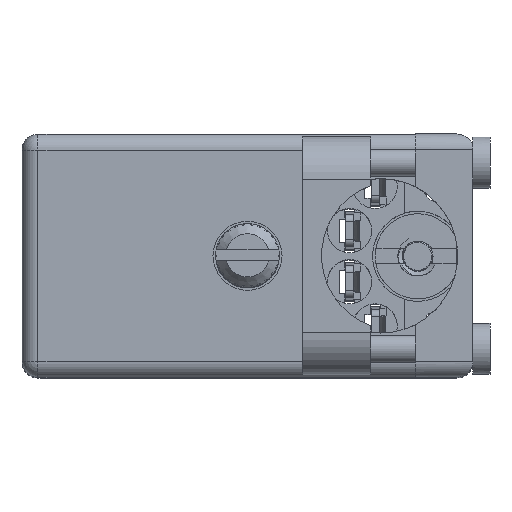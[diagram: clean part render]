
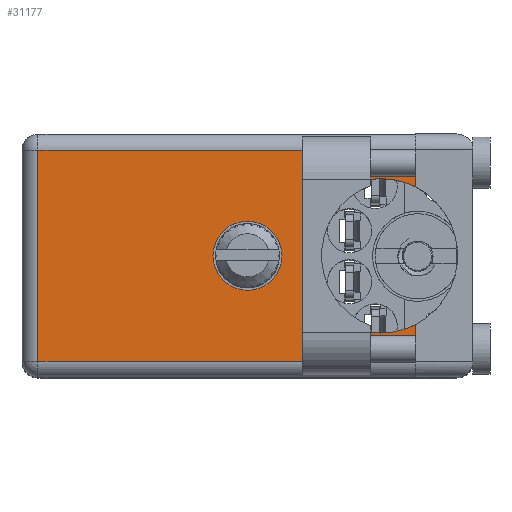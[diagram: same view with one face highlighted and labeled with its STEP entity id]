
A CAD part, top view. The second image highlights one B-rep face of the part: STEP entity #31177.
In plain terms, the highlighted face is planar.
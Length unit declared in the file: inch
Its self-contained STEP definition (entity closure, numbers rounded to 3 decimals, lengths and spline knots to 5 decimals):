
#836 = VERTEX_POINT ( 'NONE', #193161 ) ;
#1619 = CARTESIAN_POINT ( 'NONE',  ( 1.155, 0.906, -0.15471 ) ) ;
#1675 = CARTESIAN_POINT ( 'NONE',  ( 1.155, 0.906, -0.668 ) ) ;
#5758 = DIRECTION ( 'NONE',  ( 0., 0., 1. ) ) ;
#6183 = CARTESIAN_POINT ( 'NONE',  ( 1.155, 0.906, 0. ) ) ;
#8776 = CARTESIAN_POINT ( 'NONE',  ( 1.053, 0.906, -0.5845 ) ) ;
#14136 = DIRECTION ( 'NONE',  ( 0., 1., 0. ) ) ;
#14505 = ORIENTED_EDGE ( 'NONE', *, *, #89355, .T. ) ;
#15905 = VERTEX_POINT ( 'NONE', #1619 ) ;
#20903 = DIRECTION ( 'NONE',  ( 0., 0., 1. ) ) ;
#24156 = VECTOR ( 'NONE', #189563, 39.37008 ) ;
#27023 = ORIENTED_EDGE ( 'NONE', *, *, #172200, .F. ) ;
#27527 = CARTESIAN_POINT ( 'NONE',  ( 1.155, 0.906, -0.047 ) ) ;
#28790 = CARTESIAN_POINT ( 'NONE',  ( 1.053, 0.906, -0.3575 ) ) ;
#31177 = ADVANCED_FACE ( 'NONE', ( #39452, #183516 ), #131591, .T. ) ;
#31375 = EDGE_CURVE ( 'NONE', #836, #15905, #49074, .T. ) ;
#31876 = ORIENTED_EDGE ( 'NONE', *, *, #49957, .F. ) ;
#34957 = DIRECTION ( 'NONE',  ( 0., 1., 0. ) ) ;
#35433 = CIRCLE ( 'NONE', #134394, 0.227 ) ;
#38335 = DIRECTION ( 'NONE',  ( 0., 1., 0. ) ) ;
#39452 = FACE_OUTER_BOUND ( 'NONE', #113883, .T. ) ;
#41365 = VERTEX_POINT ( 'NONE', #27527 ) ;
#45925 = VECTOR ( 'NONE', #118477, 39.37008 ) ;
#46874 = VERTEX_POINT ( 'NONE', #136284 ) ;
#47317 = ORIENTED_EDGE ( 'NONE', *, *, #54023, .F. ) ;
#48261 = CARTESIAN_POINT ( 'NONE',  ( 1.053, 0.906, -0.3575 ) ) ;
#49074 = CIRCLE ( 'NONE', #132033, 0.227 ) ;
#49957 = EDGE_CURVE ( 'NONE', #15905, #41365, #113801, .T. ) ;
#51064 = CIRCLE ( 'NONE', #194340, 0.1015 ) ;
#52825 = EDGE_CURVE ( 'NONE', #46874, #169015, #164127, .T. ) ;
#53224 = ORIENTED_EDGE ( 'NONE', *, *, #100716, .T. ) ;
#53752 = DIRECTION ( 'NONE',  ( 0., 0., 1. ) ) ;
#54023 = EDGE_CURVE ( 'NONE', #106126, #138339, #51064, .T. ) ;
#63865 = AXIS2_PLACEMENT_3D ( 'NONE', #70549, #38335, #53752 ) ;
#64780 = CARTESIAN_POINT ( 'NONE',  ( 1.155, 0.906, -0.047 ) ) ;
#70549 = CARTESIAN_POINT ( 'NONE',  ( 0., 0.906, -0.715 ) ) ;
#72922 = LINE ( 'NONE', #169577, #183416 ) ;
#74742 = ORIENTED_EDGE ( 'NONE', *, *, #172307, .T. ) ;
#79443 = VECTOR ( 'NONE', #91488, 39.37008 ) ;
#79704 = CARTESIAN_POINT ( 'NONE',  ( 0.6625, 0.906, -0.459 ) ) ;
#87157 = EDGE_LOOP ( 'NONE', ( #27023, #47317 ) ) ;
#89355 = EDGE_CURVE ( 'NONE', #160134, #141707, #72922, .T. ) ;
#89523 = CARTESIAN_POINT ( 'NONE',  ( 0.6625, 0.906, -0.3575 ) ) ;
#91488 = DIRECTION ( 'NONE',  ( -1., 0., 0. ) ) ;
#91901 = ORIENTED_EDGE ( 'NONE', *, *, #52825, .F. ) ;
#92807 = CARTESIAN_POINT ( 'NONE',  ( 0., 0.906, -0.668 ) ) ;
#97363 = DIRECTION ( 'NONE',  ( 0., 0., 1. ) ) ;
#98261 = DIRECTION ( 'NONE',  ( 0., 1., 0. ) ) ;
#100716 = EDGE_CURVE ( 'NONE', #141707, #41365, #161063, .T. ) ;
#101502 = CARTESIAN_POINT ( 'NONE',  ( 0.047, 0.906, -0.047 ) ) ;
#105971 = DIRECTION ( 'NONE',  ( 0., 0., 1. ) ) ;
#106126 = VERTEX_POINT ( 'NONE', #79704 ) ;
#113801 = LINE ( 'NONE', #6183, #154682 ) ;
#113883 = EDGE_LOOP ( 'NONE', ( #169012, #74742, #14505, #53224, #31876, #192184, #127683, #91901 ) ) ;
#114638 = AXIS2_PLACEMENT_3D ( 'NONE', #89523, #134507, #194265 ) ;
#118477 = DIRECTION ( 'NONE',  ( 0., 0., 1. ) ) ;
#126074 = DIRECTION ( 'NONE',  ( 0., 1., 0. ) ) ;
#126608 = EDGE_CURVE ( 'NONE', #169015, #836, #35433, .T. ) ;
#127683 = ORIENTED_EDGE ( 'NONE', *, *, #126608, .F. ) ;
#131591 = PLANE ( 'NONE',  #63865 ) ;
#132033 = AXIS2_PLACEMENT_3D ( 'NONE', #48261, #126074, #171063 ) ;
#134394 = AXIS2_PLACEMENT_3D ( 'NONE', #28790, #14136, #105971 ) ;
#134507 = DIRECTION ( 'NONE',  ( 0., 1., 0. ) ) ;
#136284 = CARTESIAN_POINT ( 'NONE',  ( 1.155, 0.906, -0.56029 ) ) ;
#138339 = VERTEX_POINT ( 'NONE', #154897 ) ;
#139517 = CIRCLE ( 'NONE', #114638, 0.1015 ) ;
#141707 = VERTEX_POINT ( 'NONE', #101502 ) ;
#143038 = CARTESIAN_POINT ( 'NONE',  ( 1.053, 0.906, -0.3575 ) ) ;
#143301 = CARTESIAN_POINT ( 'NONE',  ( 0.6625, 0.906, -0.3575 ) ) ;
#149118 = LINE ( 'NONE', #92807, #79443 ) ;
#154682 = VECTOR ( 'NONE', #20903, 39.37008 ) ;
#154897 = CARTESIAN_POINT ( 'NONE',  ( 0.6625, 0.906, -0.256 ) ) ;
#159346 = AXIS2_PLACEMENT_3D ( 'NONE', #143038, #34957, #97363 ) ;
#160134 = VERTEX_POINT ( 'NONE', #198026 ) ;
#161063 = LINE ( 'NONE', #64780, #24156 ) ;
#161597 = EDGE_CURVE ( 'NONE', #173323, #46874, #170693, .T. ) ;
#164127 = CIRCLE ( 'NONE', #159346, 0.227 ) ;
#169012 = ORIENTED_EDGE ( 'NONE', *, *, #161597, .F. ) ;
#169015 = VERTEX_POINT ( 'NONE', #8776 ) ;
#169577 = CARTESIAN_POINT ( 'NONE',  ( 0.047, 0.906, -0.715 ) ) ;
#170693 = LINE ( 'NONE', #178916, #45925 ) ;
#171063 = DIRECTION ( 'NONE',  ( 0., 0., 1. ) ) ;
#172200 = EDGE_CURVE ( 'NONE', #138339, #106126, #139517, .T. ) ;
#172307 = EDGE_CURVE ( 'NONE', #173323, #160134, #149118, .T. ) ;
#173323 = VERTEX_POINT ( 'NONE', #1675 ) ;
#178916 = CARTESIAN_POINT ( 'NONE',  ( 1.155, 0.906, 0. ) ) ;
#183416 = VECTOR ( 'NONE', #185052, 39.37008 ) ;
#183516 = FACE_BOUND ( 'NONE', #87157, .T. ) ;
#185052 = DIRECTION ( 'NONE',  ( 0., 0., 1. ) ) ;
#189563 = DIRECTION ( 'NONE',  ( 1., 0., 0. ) ) ;
#192184 = ORIENTED_EDGE ( 'NONE', *, *, #31375, .F. ) ;
#193161 = CARTESIAN_POINT ( 'NONE',  ( 1.053, 0.906, -0.1305 ) ) ;
#194265 = DIRECTION ( 'NONE',  ( 0., 0., 1. ) ) ;
#194340 = AXIS2_PLACEMENT_3D ( 'NONE', #143301, #98261, #5758 ) ;
#198026 = CARTESIAN_POINT ( 'NONE',  ( 0.047, 0.906, -0.668 ) ) ;
